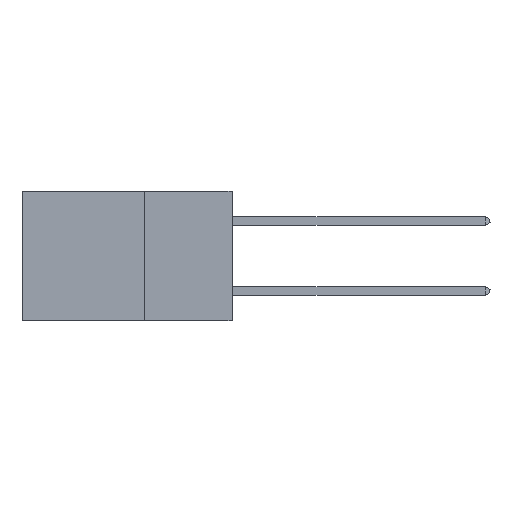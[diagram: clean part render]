
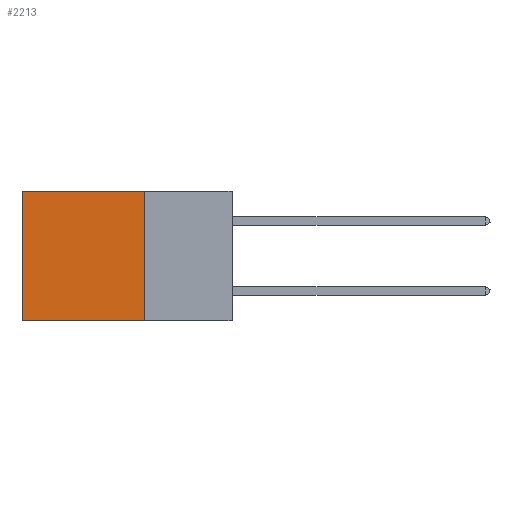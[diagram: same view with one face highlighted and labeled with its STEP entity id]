
A CAD part, left-side view. The second image highlights one B-rep face of the part: STEP entity #2213.
In plain terms, the highlighted planar face has unit normal (-1, 0, 0).
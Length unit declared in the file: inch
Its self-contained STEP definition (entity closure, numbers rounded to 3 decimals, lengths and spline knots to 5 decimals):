
#874 = CARTESIAN_POINT ( 'NONE',  ( 0.2875, 0.25, 0. ) ) ;
#1114 = CARTESIAN_POINT ( 'NONE',  ( 0.2875, 0.25, -0.37 ) ) ;
#1220 = EDGE_CURVE ( 'NONE', #1926, #24180, #8565, .T. ) ;
#1926 = VERTEX_POINT ( 'NONE', #16843 ) ;
#2213 = ADVANCED_FACE ( 'NONE', ( #28603 ), #15381, .F. ) ;
#3215 = VECTOR ( 'NONE', #21534, 39.37008 ) ;
#3397 = DIRECTION ( 'NONE',  ( 1., 0., 0. ) ) ;
#4880 = ORIENTED_EDGE ( 'NONE', *, *, #16690, .F. ) ;
#5526 = LINE ( 'NONE', #1114, #10446 ) ;
#6428 = LINE ( 'NONE', #6430, #18331 ) ;
#6430 = CARTESIAN_POINT ( 'NONE',  ( 0.2875, 0.25, 0. ) ) ;
#8565 = LINE ( 'NONE', #11991, #21196 ) ;
#8569 = EDGE_CURVE ( 'NONE', #24180, #11620, #9683, .T. ) ;
#9683 = LINE ( 'NONE', #19128, #3215 ) ;
#10446 = VECTOR ( 'NONE', #20372, 39.37008 ) ;
#10881 = CARTESIAN_POINT ( 'NONE',  ( 0.2875, 0.6, 0. ) ) ;
#11620 = VERTEX_POINT ( 'NONE', #23898 ) ;
#11991 = CARTESIAN_POINT ( 'NONE',  ( 0.2875, 0.25, 0. ) ) ;
#12132 = AXIS2_PLACEMENT_3D ( 'NONE', #874, #3397, #20126 ) ;
#12598 = ORIENTED_EDGE ( 'NONE', *, *, #1220, .T. ) ;
#14375 = DIRECTION ( 'NONE',  ( 0., 1., 0. ) ) ;
#14435 = EDGE_LOOP ( 'NONE', ( #26327, #4880, #15910, #12598 ) ) ;
#14579 = EDGE_CURVE ( 'NONE', #1926, #22710, #6428, .T. ) ;
#15381 = PLANE ( 'NONE',  #12132 ) ;
#15910 = ORIENTED_EDGE ( 'NONE', *, *, #14579, .F. ) ;
#16690 = EDGE_CURVE ( 'NONE', #22710, #11620, #5526, .T. ) ;
#16843 = CARTESIAN_POINT ( 'NONE',  ( 0.2875, 0.25, 0. ) ) ;
#18331 = VECTOR ( 'NONE', #25462, 39.37008 ) ;
#19128 = CARTESIAN_POINT ( 'NONE',  ( 0.2875, 0.6, 0. ) ) ;
#20126 = DIRECTION ( 'NONE',  ( 0., 0., -1. ) ) ;
#20372 = DIRECTION ( 'NONE',  ( 0., 1., 0. ) ) ;
#21196 = VECTOR ( 'NONE', #14375, 39.37008 ) ;
#21534 = DIRECTION ( 'NONE',  ( 0., 0., -1. ) ) ;
#22710 = VERTEX_POINT ( 'NONE', #30707 ) ;
#23898 = CARTESIAN_POINT ( 'NONE',  ( 0.2875, 0.6, -0.37 ) ) ;
#24180 = VERTEX_POINT ( 'NONE', #10881 ) ;
#25462 = DIRECTION ( 'NONE',  ( 0., 0., -1. ) ) ;
#26327 = ORIENTED_EDGE ( 'NONE', *, *, #8569, .T. ) ;
#28603 = FACE_OUTER_BOUND ( 'NONE', #14435, .T. ) ;
#30707 = CARTESIAN_POINT ( 'NONE',  ( 0.2875, 0.25, -0.37 ) ) ;
